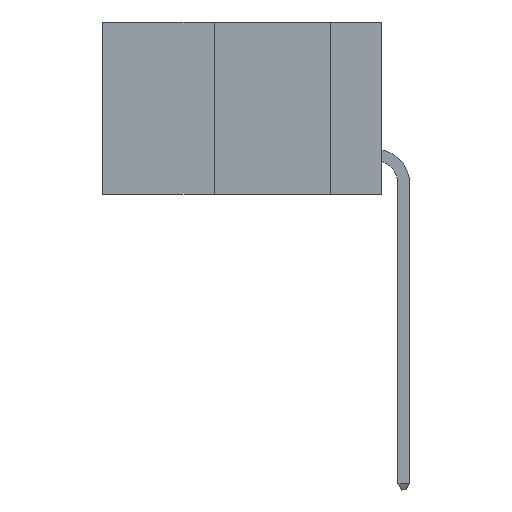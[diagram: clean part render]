
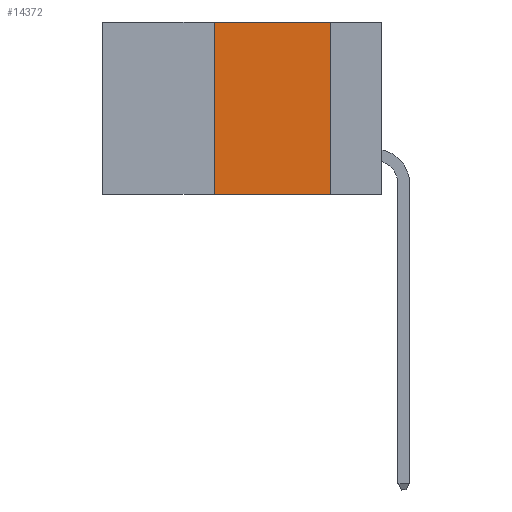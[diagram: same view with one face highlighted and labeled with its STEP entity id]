
A CAD part, left-side view. The second image highlights one B-rep face of the part: STEP entity #14372.
In plain terms, the highlighted planar face has unit normal (-1, 0, 0).
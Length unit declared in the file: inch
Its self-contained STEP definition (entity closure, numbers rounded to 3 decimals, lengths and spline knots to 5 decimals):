
#841 = DIRECTION ( 'NONE',  ( 1., 0., 0. ) ) ;
#1890 = CARTESIAN_POINT ( 'NONE',  ( 0., 0.11, -0.37 ) ) ;
#2165 = CARTESIAN_POINT ( 'NONE',  ( 0., 0.36, 0. ) ) ;
#2753 = LINE ( 'NONE', #7512, #9139 ) ;
#2961 = VECTOR ( 'NONE', #4483, 39.37008 ) ;
#3866 = VERTEX_POINT ( 'NONE', #18397 ) ;
#4483 = DIRECTION ( 'NONE',  ( 0., 0., -1. ) ) ;
#5366 = LINE ( 'NONE', #16122, #2961 ) ;
#5571 = ORIENTED_EDGE ( 'NONE', *, *, #8856, .F. ) ;
#7512 = CARTESIAN_POINT ( 'NONE',  ( 0., 0.6, 0. ) ) ;
#8030 = EDGE_CURVE ( 'NONE', #20136, #12588, #14534, .T. ) ;
#8856 = EDGE_CURVE ( 'NONE', #9621, #12588, #5366, .T. ) ;
#9117 = EDGE_CURVE ( 'NONE', #20136, #3866, #17779, .T. ) ;
#9139 = VECTOR ( 'NONE', #17203, 39.37008 ) ;
#9621 = VERTEX_POINT ( 'NONE', #17424 ) ;
#10696 = DIRECTION ( 'NONE',  ( 0., 0., -1. ) ) ;
#12185 = ORIENTED_EDGE ( 'NONE', *, *, #9117, .F. ) ;
#12468 = CARTESIAN_POINT ( 'NONE',  ( 0., 0.6, 0. ) ) ;
#12588 = VERTEX_POINT ( 'NONE', #1890 ) ;
#14145 = DIRECTION ( 'NONE',  ( 0., 0., 1. ) ) ;
#14372 = ADVANCED_FACE ( 'NONE', ( #21306 ), #22056, .F. ) ;
#14534 = LINE ( 'NONE', #15774, #21190 ) ;
#15677 = VECTOR ( 'NONE', #14145, 39.37008 ) ;
#15774 = CARTESIAN_POINT ( 'NONE',  ( 0., 0.6, -0.37 ) ) ;
#16122 = CARTESIAN_POINT ( 'NONE',  ( 0., 0.11, 0. ) ) ;
#16940 = AXIS2_PLACEMENT_3D ( 'NONE', #12468, #841, #10696 ) ;
#17036 = EDGE_LOOP ( 'NONE', ( #5571, #24017, #12185, #21328 ) ) ;
#17203 = DIRECTION ( 'NONE',  ( 0., -1., 0. ) ) ;
#17424 = CARTESIAN_POINT ( 'NONE',  ( 0., 0.11, 0. ) ) ;
#17779 = LINE ( 'NONE', #2165, #15677 ) ;
#18397 = CARTESIAN_POINT ( 'NONE',  ( 0., 0.36, 0. ) ) ;
#18799 = EDGE_CURVE ( 'NONE', #3866, #9621, #2753, .T. ) ;
#19588 = DIRECTION ( 'NONE',  ( 0., -1., 0. ) ) ;
#20136 = VERTEX_POINT ( 'NONE', #24745 ) ;
#21190 = VECTOR ( 'NONE', #19588, 39.37008 ) ;
#21306 = FACE_OUTER_BOUND ( 'NONE', #17036, .T. ) ;
#21328 = ORIENTED_EDGE ( 'NONE', *, *, #8030, .T. ) ;
#22056 = PLANE ( 'NONE',  #16940 ) ;
#24017 = ORIENTED_EDGE ( 'NONE', *, *, #18799, .F. ) ;
#24745 = CARTESIAN_POINT ( 'NONE',  ( 0., 0.36, -0.37 ) ) ;
